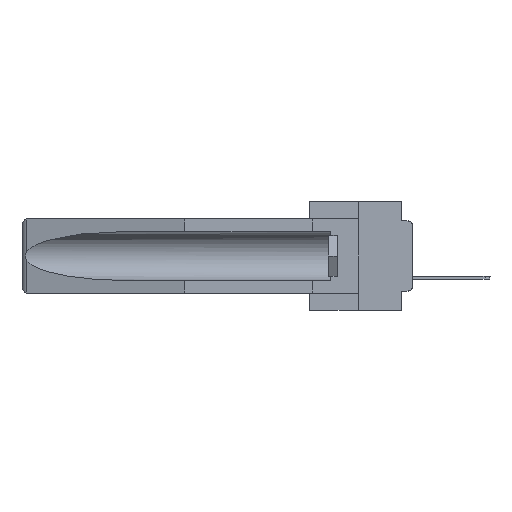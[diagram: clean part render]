
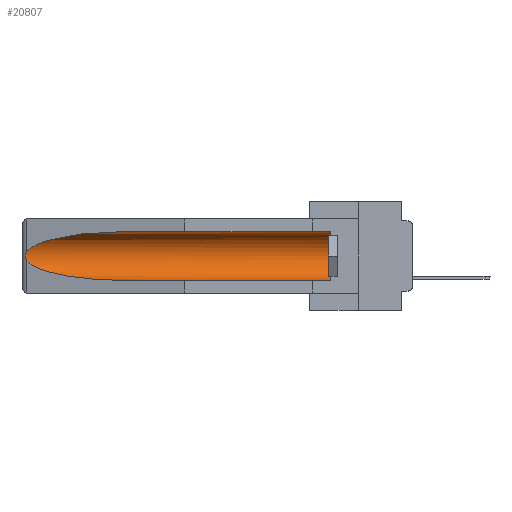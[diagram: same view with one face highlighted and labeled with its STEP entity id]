
A CAD part, left-side view. The second image highlights one B-rep face of the part: STEP entity #20807.
In plain terms, the highlighted cylindrical face has radius 2.857 mm (diameter 5.715 mm), a partial arc.
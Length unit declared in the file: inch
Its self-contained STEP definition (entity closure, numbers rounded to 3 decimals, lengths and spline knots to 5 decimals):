
#32 = EDGE_CURVE ( 'NONE', #5700, #24859, #21611, .T. ) ;
#81 = CARTESIAN_POINT ( 'NONE',  ( 0.155, 0.126, -0.059 ) ) ;
#356 = EDGE_CURVE ( 'NONE', #33888, #5700, #2956, .T. ) ;
#1433 = CARTESIAN_POINT ( 'NONE',  ( 0.26537, 1.52718, -0.19328 ) ) ;
#1921 = DIRECTION ( 'NONE',  ( 0., 1., 0. ) ) ;
#2694 = LINE ( 'NONE', #31007, #25746 ) ;
#2956 = LINE ( 'NONE', #22567, #23964 ) ;
#3925 = CARTESIAN_POINT ( 'NONE',  ( 0.2675, 1.53308, -0.16763 ) ) ;
#4443 = CARTESIAN_POINT ( 'NONE',  ( 0.155, 0.126, -0.284 ) ) ;
#5700 = VERTEX_POINT ( 'NONE', #9720 ) ;
#6015 = VERTEX_POINT ( 'NONE', #4443 ) ;
#6178 = DIRECTION ( 'NONE',  ( 0., 1., 0. ) ) ;
#6458 = CARTESIAN_POINT ( 'NONE',  ( 0.26537, 1.52718, -0.14972 ) ) ;
#6515 = CARTESIAN_POINT ( 'NONE',  ( 0.25451, 1.48313, -0.24835 ) ) ;
#6586 = CARTESIAN_POINT ( 'NONE',  ( 0.26597, 1.5296, -0.19026 ) ) ;
#6613 = AXIS2_PLACEMENT_3D ( 'NONE', #20364, #1921, #34862 ) ;
#8100 = ORIENTED_EDGE ( 'NONE', *, *, #14983, .T. ) ;
#8881 = B_SPLINE_CURVE_WITH_KNOTS ( 'NONE', 3,
 ( #6458, #8961, #28310, #22938, #3925, #31048, #14694, #14804, #6586, #9328 ),
 .UNSPECIFIED., .F., .F.,
 ( 4, 2, 2, 2, 4 ),
 ( 0., 0.00029, 0.00058, 0.00087, 0.00117 ),
 .UNSPECIFIED. ) ;
#8961 = CARTESIAN_POINT ( 'NONE',  ( 0.26597, 1.52961, -0.15275 ) ) ;
#9327 = CARTESIAN_POINT ( 'NONE',  ( 0.26537, 1.52718, -0.14972 ) ) ;
#9328 = CARTESIAN_POINT ( 'NONE',  ( 0.26537, 1.52718, -0.19328 ) ) ;
#9597 = VERTEX_POINT ( 'NONE', #27458 ) ;
#9720 = CARTESIAN_POINT ( 'NONE',  ( 0.155, 1.07973, -0.059 ) ) ;
#11829 = DIRECTION ( 'NONE',  ( 0., 1., 0. ) ) ;
#14694 = CARTESIAN_POINT ( 'NONE',  ( 0.2673, 1.53269, -0.17917 ) ) ;
#14736 = CYLINDRICAL_SURFACE ( 'NONE', #6613, 0.1125 ) ;
#14804 = CARTESIAN_POINT ( 'NONE',  ( 0.26655, 1.53094, -0.18657 ) ) ;
#14983 = EDGE_CURVE ( 'NONE', #9597, #27215, #35452, .T. ) ;
#15443 = DIRECTION ( 'NONE',  ( 0., 0., 1. ) ) ;
#17623 = EDGE_LOOP ( 'NONE', ( #27101, #18856, #8100, #35250, #28510, #26968 ) ) ;
#18212 = CARTESIAN_POINT ( 'NONE',  ( 0.21114, 1.30732, -0.059 ) ) ;
#18456 = CARTESIAN_POINT ( 'NONE',  ( 0.155, 1.07973, -0.059 ) ) ;
#18776 = CARTESIAN_POINT ( 'NONE',  ( 0.155, 1.07973, -0.284 ) ) ;
#18822 = EDGE_CURVE ( 'NONE', #24859, #9597, #8881, .T. ) ;
#18856 = ORIENTED_EDGE ( 'NONE', *, *, #18822, .T. ) ;
#20364 = CARTESIAN_POINT ( 'NONE',  ( 0.155, -0.30754, -0.1715 ) ) ;
#20807 = ADVANCED_FACE ( 'NONE', ( #30532 ), #14736, .F. ) ;
#21611 =( BOUNDED_CURVE ( )  B_SPLINE_CURVE ( 3, ( #18456, #18212, #29427, #23728 ),
 .UNSPECIFIED., .F., .F. ) 
 B_SPLINE_CURVE_WITH_KNOTS ( ( 4, 4 ),
 ( 4.71239, 6.08839 ),
 .UNSPECIFIED. ) 
 CURVE ( )  GEOMETRIC_REPRESENTATION_ITEM ( )  RATIONAL_B_SPLINE_CURVE ( ( 1., 0.848, 0.848, 1. ) ) 
 REPRESENTATION_ITEM ( '' )  );
#21936 = EDGE_CURVE ( 'NONE', #6015, #27215, #2694, .T. ) ;
#22005 = AXIS2_PLACEMENT_3D ( 'NONE', #31573, #23451, #15443 ) ;
#22567 = CARTESIAN_POINT ( 'NONE',  ( 0.155, -0.30754, -0.059 ) ) ;
#22891 = CIRCLE ( 'NONE', #22005, 0.1125 ) ;
#22938 = CARTESIAN_POINT ( 'NONE',  ( 0.2673, 1.5327, -0.16383 ) ) ;
#23232 = CARTESIAN_POINT ( 'NONE',  ( 0.21114, 1.30732, -0.284 ) ) ;
#23451 = DIRECTION ( 'NONE',  ( 0., -1., 0. ) ) ;
#23728 = CARTESIAN_POINT ( 'NONE',  ( 0.26537, 1.52718, -0.14972 ) ) ;
#23964 = VECTOR ( 'NONE', #11829, 39.37008 ) ;
#24859 = VERTEX_POINT ( 'NONE', #9327 ) ;
#25739 = CARTESIAN_POINT ( 'NONE',  ( 0.155, 1.07973, -0.284 ) ) ;
#25746 = VECTOR ( 'NONE', #6178, 39.37008 ) ;
#26968 = ORIENTED_EDGE ( 'NONE', *, *, #356, .T. ) ;
#27101 = ORIENTED_EDGE ( 'NONE', *, *, #32, .T. ) ;
#27215 = VERTEX_POINT ( 'NONE', #18776 ) ;
#27458 = CARTESIAN_POINT ( 'NONE',  ( 0.26537, 1.52718, -0.19328 ) ) ;
#28136 = EDGE_CURVE ( 'NONE', #6015, #33888, #22891, .T. ) ;
#28310 = CARTESIAN_POINT ( 'NONE',  ( 0.26654, 1.53092, -0.15636 ) ) ;
#28510 = ORIENTED_EDGE ( 'NONE', *, *, #28136, .T. ) ;
#29427 = CARTESIAN_POINT ( 'NONE',  ( 0.25451, 1.48313, -0.09465 ) ) ;
#30532 = FACE_OUTER_BOUND ( 'NONE', #17623, .T. ) ;
#31007 = CARTESIAN_POINT ( 'NONE',  ( 0.155, -0.30754, -0.284 ) ) ;
#31048 = CARTESIAN_POINT ( 'NONE',  ( 0.2675, 1.53308, -0.17534 ) ) ;
#31573 = CARTESIAN_POINT ( 'NONE',  ( 0.155, 0.126, -0.1715 ) ) ;
#33888 = VERTEX_POINT ( 'NONE', #81 ) ;
#34862 = DIRECTION ( 'NONE',  ( 0., 0., 1. ) ) ;
#35250 = ORIENTED_EDGE ( 'NONE', *, *, #21936, .F. ) ;
#35452 =( BOUNDED_CURVE ( )  B_SPLINE_CURVE ( 3, ( #1433, #6515, #23232, #25739 ),
 .UNSPECIFIED., .F., .T. ) 
 B_SPLINE_CURVE_WITH_KNOTS ( ( 4, 4 ),
 ( 0.1948, 1.5708 ),
 .UNSPECIFIED. ) 
 CURVE ( )  GEOMETRIC_REPRESENTATION_ITEM ( )  RATIONAL_B_SPLINE_CURVE ( ( 1., 0.848, 0.848, 1. ) ) 
 REPRESENTATION_ITEM ( '' )  );
